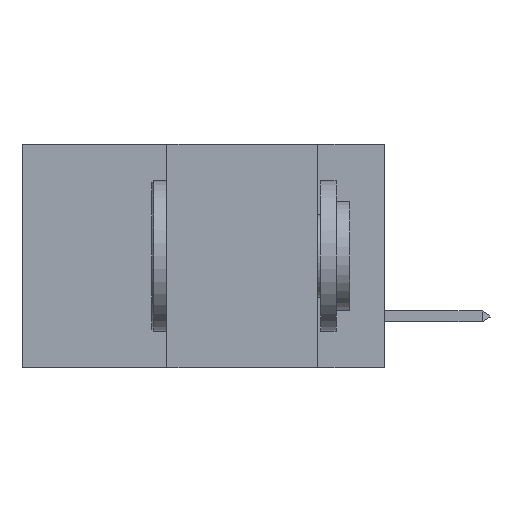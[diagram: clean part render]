
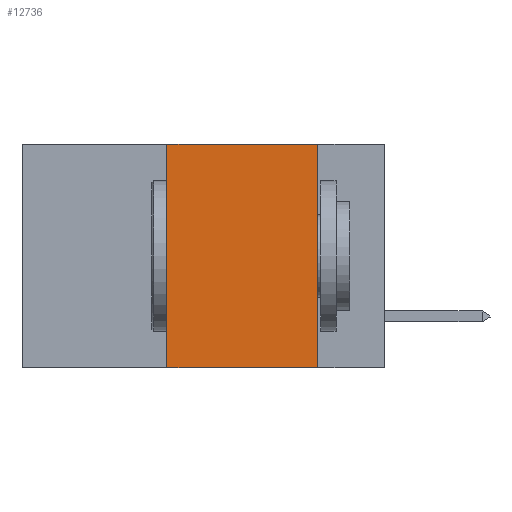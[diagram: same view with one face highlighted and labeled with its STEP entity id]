
A CAD part, left-side view. The second image highlights one B-rep face of the part: STEP entity #12736.
In plain terms, the highlighted planar face has unit normal (-1, 0, 0).
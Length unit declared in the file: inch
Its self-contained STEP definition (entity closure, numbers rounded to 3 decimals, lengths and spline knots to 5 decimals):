
#353 = CARTESIAN_POINT ( 'NONE',  ( 0., 0.36, 0. ) ) ;
#470 = LINE ( 'NONE', #8927, #1628 ) ;
#529 = DIRECTION ( 'NONE',  ( 0., 0., -1. ) ) ;
#648 = CARTESIAN_POINT ( 'NONE',  ( 0., 0.36, 0. ) ) ;
#1149 = ORIENTED_EDGE ( 'NONE', *, *, #12436, .F. ) ;
#1628 = VECTOR ( 'NONE', #529, 39.37008 ) ;
#2538 = LINE ( 'NONE', #11776, #12370 ) ;
#3174 = EDGE_CURVE ( 'NONE', #3550, #11448, #7402, .T. ) ;
#3258 = ORIENTED_EDGE ( 'NONE', *, *, #3174, .F. ) ;
#3267 = DIRECTION ( 'NONE',  ( 0., 0., -1. ) ) ;
#3368 = PLANE ( 'NONE',  #6887 ) ;
#3457 = DIRECTION ( 'NONE',  ( 0., 0., 1. ) ) ;
#3517 = CARTESIAN_POINT ( 'NONE',  ( 0., 0.36, -0.37 ) ) ;
#3550 = VERTEX_POINT ( 'NONE', #648 ) ;
#3954 = ORIENTED_EDGE ( 'NONE', *, *, #4935, .F. ) ;
#3960 = EDGE_CURVE ( 'NONE', #4014, #5124, #2538, .T. ) ;
#4014 = VERTEX_POINT ( 'NONE', #3517 ) ;
#4291 = LINE ( 'NONE', #353, #4772 ) ;
#4345 = DIRECTION ( 'NONE',  ( 1., 0., 0. ) ) ;
#4645 = VECTOR ( 'NONE', #7308, 39.37008 ) ;
#4772 = VECTOR ( 'NONE', #3457, 39.37008 ) ;
#4935 = EDGE_CURVE ( 'NONE', #4014, #3550, #4291, .T. ) ;
#5124 = VERTEX_POINT ( 'NONE', #12489 ) ;
#6270 = CARTESIAN_POINT ( 'NONE',  ( 0., 0.6, 0. ) ) ;
#6887 = AXIS2_PLACEMENT_3D ( 'NONE', #10531, #4345, #3267 ) ;
#7308 = DIRECTION ( 'NONE',  ( 0., -1., 0. ) ) ;
#7402 = LINE ( 'NONE', #6270, #4645 ) ;
#7527 = ORIENTED_EDGE ( 'NONE', *, *, #3960, .T. ) ;
#7765 = DIRECTION ( 'NONE',  ( 0., -1., 0. ) ) ;
#8927 = CARTESIAN_POINT ( 'NONE',  ( 0., 0.11, 0. ) ) ;
#10347 = CARTESIAN_POINT ( 'NONE',  ( 0., 0.11, 0. ) ) ;
#10531 = CARTESIAN_POINT ( 'NONE',  ( 0., 0.6, 0. ) ) ;
#11448 = VERTEX_POINT ( 'NONE', #10347 ) ;
#11757 = FACE_OUTER_BOUND ( 'NONE', #13362, .T. ) ;
#11776 = CARTESIAN_POINT ( 'NONE',  ( 0., 0.6, -0.37 ) ) ;
#12370 = VECTOR ( 'NONE', #7765, 39.37008 ) ;
#12436 = EDGE_CURVE ( 'NONE', #11448, #5124, #470, .T. ) ;
#12489 = CARTESIAN_POINT ( 'NONE',  ( 0., 0.11, -0.37 ) ) ;
#12736 = ADVANCED_FACE ( 'NONE', ( #11757 ), #3368, .F. ) ;
#13362 = EDGE_LOOP ( 'NONE', ( #1149, #3258, #3954, #7527 ) ) ;
